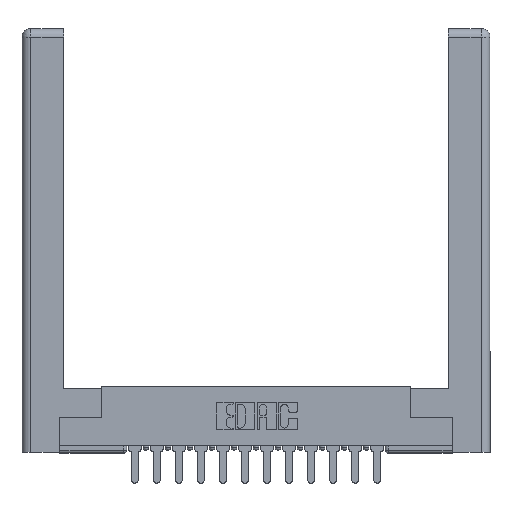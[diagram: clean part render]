
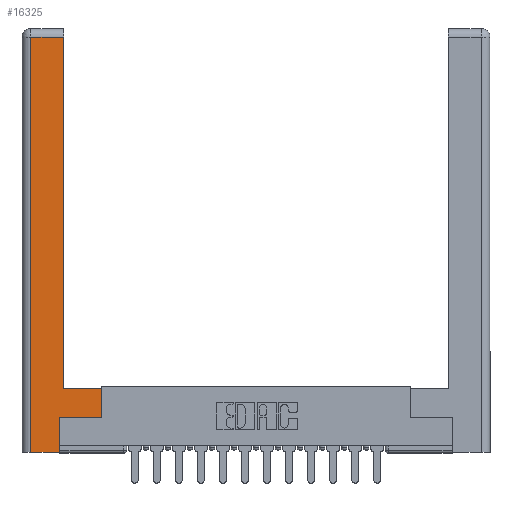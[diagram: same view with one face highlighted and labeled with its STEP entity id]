
A CAD part, top view. The second image highlights one B-rep face of the part: STEP entity #16325.
In plain terms, the highlighted planar face has unit normal (0, 0, 1).
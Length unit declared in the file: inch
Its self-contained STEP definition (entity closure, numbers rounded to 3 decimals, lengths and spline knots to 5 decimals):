
#140 = EDGE_CURVE ( 'NONE', #153, #4868, #4602, .T. ) ;
#153 = VERTEX_POINT ( 'NONE', #1687 ) ;
#219 = FACE_OUTER_BOUND ( 'NONE', #14799, .T. ) ;
#459 = EDGE_CURVE ( 'NONE', #7598, #10260, #2515, .T. ) ;
#753 = CARTESIAN_POINT ( 'NONE',  ( 0.0615, 0., 0. ) ) ;
#938 = VERTEX_POINT ( 'NONE', #11940 ) ;
#1629 = EDGE_CURVE ( 'NONE', #10260, #938, #16706, .T. ) ;
#1687 = CARTESIAN_POINT ( 'NONE',  ( 0.0615, 2.94, 0. ) ) ;
#2046 = VECTOR ( 'NONE', #3070, 39.37008 ) ;
#2092 = CARTESIAN_POINT ( 'NONE',  ( 0.265, 0.245, 0. ) ) ;
#2137 = VERTEX_POINT ( 'NONE', #12046 ) ;
#2350 = CARTESIAN_POINT ( 'NONE',  ( 0.565, 0.245, 0. ) ) ;
#2515 = LINE ( 'NONE', #2766, #16209 ) ;
#2766 = CARTESIAN_POINT ( 'NONE',  ( 0.265, 0.245, 0. ) ) ;
#3040 = VECTOR ( 'NONE', #3816, 39.37008 ) ;
#3070 = DIRECTION ( 'NONE',  ( 1., 0., 0. ) ) ;
#3816 = DIRECTION ( 'NONE',  ( 0., 1., 0. ) ) ;
#4576 = VECTOR ( 'NONE', #5553, 39.37008 ) ;
#4579 = ORIENTED_EDGE ( 'NONE', *, *, #140, .T. ) ;
#4602 = LINE ( 'NONE', #5890, #8632 ) ;
#4756 = CARTESIAN_POINT ( 'NONE',  ( 0.295, 0.45, 0. ) ) ;
#4868 = VERTEX_POINT ( 'NONE', #753 ) ;
#5085 = EDGE_CURVE ( 'NONE', #13143, #2137, #5959, .T. ) ;
#5251 = ORIENTED_EDGE ( 'NONE', *, *, #1629, .T. ) ;
#5469 = CARTESIAN_POINT ( 'NONE',  ( 0., 0., 0. ) ) ;
#5553 = DIRECTION ( 'NONE',  ( -1., 0., 0. ) ) ;
#5890 = CARTESIAN_POINT ( 'NONE',  ( 0.0615, 0., 0. ) ) ;
#5959 = LINE ( 'NONE', #4756, #4576 ) ;
#6254 = CARTESIAN_POINT ( 'NONE',  ( 0.565, 0.45, 0. ) ) ;
#6768 = DIRECTION ( 'NONE',  ( 0., 0., -1. ) ) ;
#6839 = VECTOR ( 'NONE', #7616, 39.37008 ) ;
#7080 = ORIENTED_EDGE ( 'NONE', *, *, #5085, .T. ) ;
#7293 = LINE ( 'NONE', #14924, #2046 ) ;
#7598 = VERTEX_POINT ( 'NONE', #9110 ) ;
#7616 = DIRECTION ( 'NONE',  ( 1., 0., 0. ) ) ;
#7680 = EDGE_CURVE ( 'NONE', #4868, #7598, #7293, .T. ) ;
#7789 = LINE ( 'NONE', #16629, #3040 ) ;
#7887 = DIRECTION ( 'NONE',  ( 0., 1., 0. ) ) ;
#8166 = ORIENTED_EDGE ( 'NONE', *, *, #7680, .T. ) ;
#8356 = EDGE_CURVE ( 'NONE', #938, #13143, #13020, .T. ) ;
#8632 = VECTOR ( 'NONE', #10884, 39.37008 ) ;
#8796 = EDGE_CURVE ( 'NONE', #2137, #13301, #7789, .T. ) ;
#8998 = ORIENTED_EDGE ( 'NONE', *, *, #9896, .T. ) ;
#9110 = CARTESIAN_POINT ( 'NONE',  ( 0.265, 0., 0. ) ) ;
#9438 = DIRECTION ( 'NONE',  ( -1., 0., 0. ) ) ;
#9896 = EDGE_CURVE ( 'NONE', #13301, #153, #12350, .T. ) ;
#10260 = VERTEX_POINT ( 'NONE', #2092 ) ;
#10290 = ORIENTED_EDGE ( 'NONE', *, *, #8356, .T. ) ;
#10884 = DIRECTION ( 'NONE',  ( 0., -1., 0. ) ) ;
#11561 = VECTOR ( 'NONE', #7887, 39.37008 ) ;
#11940 = CARTESIAN_POINT ( 'NONE',  ( 0.565, 0.245, 0. ) ) ;
#12046 = CARTESIAN_POINT ( 'NONE',  ( 0.295, 0.45, 0. ) ) ;
#12104 = PLANE ( 'NONE',  #15677 ) ;
#12350 = LINE ( 'NONE', #12523, #14544 ) ;
#12523 = CARTESIAN_POINT ( 'NONE',  ( 0.0615, 2.94, 0. ) ) ;
#13020 = LINE ( 'NONE', #6254, #11561 ) ;
#13143 = VERTEX_POINT ( 'NONE', #14178 ) ;
#13301 = VERTEX_POINT ( 'NONE', #13391 ) ;
#13391 = CARTESIAN_POINT ( 'NONE',  ( 0.295, 2.94, 0. ) ) ;
#13965 = DIRECTION ( 'NONE',  ( -1., 0., 0. ) ) ;
#14178 = CARTESIAN_POINT ( 'NONE',  ( 0.565, 0.45, 0. ) ) ;
#14541 = DIRECTION ( 'NONE',  ( 0., 1., 0. ) ) ;
#14544 = VECTOR ( 'NONE', #13965, 39.37008 ) ;
#14799 = EDGE_LOOP ( 'NONE', ( #16092, #8998, #4579, #8166, #15404, #5251, #10290, #7080 ) ) ;
#14924 = CARTESIAN_POINT ( 'NONE',  ( 0.265, 0., 0. ) ) ;
#15404 = ORIENTED_EDGE ( 'NONE', *, *, #459, .T. ) ;
#15677 = AXIS2_PLACEMENT_3D ( 'NONE', #5469, #6768, #9438 ) ;
#16092 = ORIENTED_EDGE ( 'NONE', *, *, #8796, .T. ) ;
#16209 = VECTOR ( 'NONE', #14541, 39.37008 ) ;
#16325 = ADVANCED_FACE ( 'NONE', ( #219 ), #12104, .F. ) ;
#16629 = CARTESIAN_POINT ( 'NONE',  ( 0.295, 3., 0. ) ) ;
#16706 = LINE ( 'NONE', #2350, #6839 ) ;
